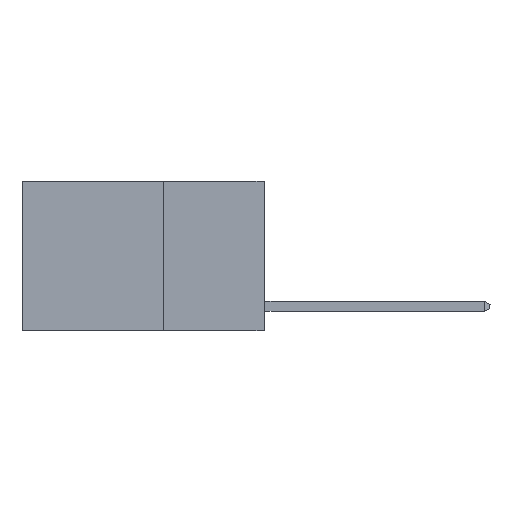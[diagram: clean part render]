
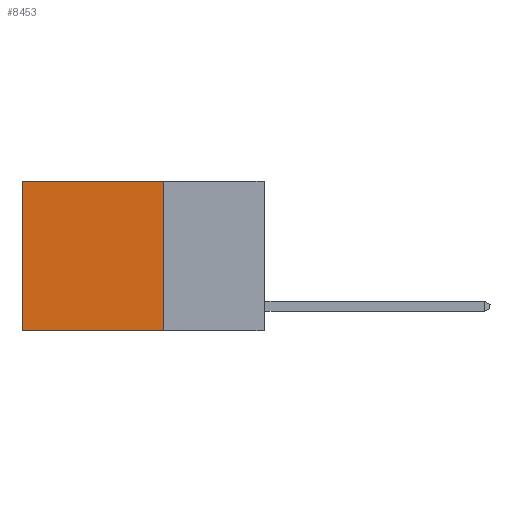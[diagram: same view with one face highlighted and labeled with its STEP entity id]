
A CAD part, left-side view. The second image highlights one B-rep face of the part: STEP entity #8453.
In plain terms, the highlighted planar face has unit normal (-1, 0, 0).
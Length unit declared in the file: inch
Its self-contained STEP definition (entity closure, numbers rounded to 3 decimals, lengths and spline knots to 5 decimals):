
#901 = DIRECTION ( 'NONE',  ( 0., 0., -1. ) ) ;
#2330 = VECTOR ( 'NONE', #9114, 39.37008 ) ;
#3414 = EDGE_CURVE ( 'NONE', #11716, #14574, #15453, .T. ) ;
#3428 = DIRECTION ( 'NONE',  ( 0., 0., -1. ) ) ;
#4410 = LINE ( 'NONE', #11900, #2330 ) ;
#5860 = DIRECTION ( 'NONE',  ( 0., 1., 0. ) ) ;
#6050 = LINE ( 'NONE', #14969, #13320 ) ;
#6426 = CARTESIAN_POINT ( 'NONE',  ( 0.2625, 0.25, 0. ) ) ;
#7691 = EDGE_LOOP ( 'NONE', ( #8396, #17881, #8782, #14144 ) ) ;
#8182 = VECTOR ( 'NONE', #18227, 39.37008 ) ;
#8396 = ORIENTED_EDGE ( 'NONE', *, *, #3414, .T. ) ;
#8453 = ADVANCED_FACE ( 'NONE', ( #8475 ), #11667, .F. ) ;
#8475 = FACE_OUTER_BOUND ( 'NONE', #7691, .T. ) ;
#8613 = CARTESIAN_POINT ( 'NONE',  ( 0.2625, 0.6, -0.37 ) ) ;
#8782 = ORIENTED_EDGE ( 'NONE', *, *, #9335, .F. ) ;
#9023 = CARTESIAN_POINT ( 'NONE',  ( 0.2625, 0.25, -0.37 ) ) ;
#9114 = DIRECTION ( 'NONE',  ( 0., 0., -1. ) ) ;
#9335 = EDGE_CURVE ( 'NONE', #10484, #13308, #4410, .T. ) ;
#10285 = AXIS2_PLACEMENT_3D ( 'NONE', #14577, #17781, #901 ) ;
#10484 = VERTEX_POINT ( 'NONE', #6426 ) ;
#11667 = PLANE ( 'NONE',  #10285 ) ;
#11716 = VERTEX_POINT ( 'NONE', #13660 ) ;
#11900 = CARTESIAN_POINT ( 'NONE',  ( 0.2625, 0.25, 0. ) ) ;
#12419 = CARTESIAN_POINT ( 'NONE',  ( 0.2625, 0.6, 0. ) ) ;
#13308 = VERTEX_POINT ( 'NONE', #19342 ) ;
#13320 = VECTOR ( 'NONE', #5860, 39.37008 ) ;
#13660 = CARTESIAN_POINT ( 'NONE',  ( 0.2625, 0.6, 0. ) ) ;
#13798 = LINE ( 'NONE', #9023, #8182 ) ;
#14144 = ORIENTED_EDGE ( 'NONE', *, *, #15606, .T. ) ;
#14574 = VERTEX_POINT ( 'NONE', #8613 ) ;
#14577 = CARTESIAN_POINT ( 'NONE',  ( 0.2625, 0.25, 0. ) ) ;
#14711 = EDGE_CURVE ( 'NONE', #13308, #14574, #13798, .T. ) ;
#14969 = CARTESIAN_POINT ( 'NONE',  ( 0.2625, 0.25, 0. ) ) ;
#15453 = LINE ( 'NONE', #12419, #15918 ) ;
#15606 = EDGE_CURVE ( 'NONE', #10484, #11716, #6050, .T. ) ;
#15918 = VECTOR ( 'NONE', #3428, 39.37008 ) ;
#17781 = DIRECTION ( 'NONE',  ( 1., 0., 0. ) ) ;
#17881 = ORIENTED_EDGE ( 'NONE', *, *, #14711, .F. ) ;
#18227 = DIRECTION ( 'NONE',  ( 0., 1., 0. ) ) ;
#19342 = CARTESIAN_POINT ( 'NONE',  ( 0.2625, 0.25, -0.37 ) ) ;
